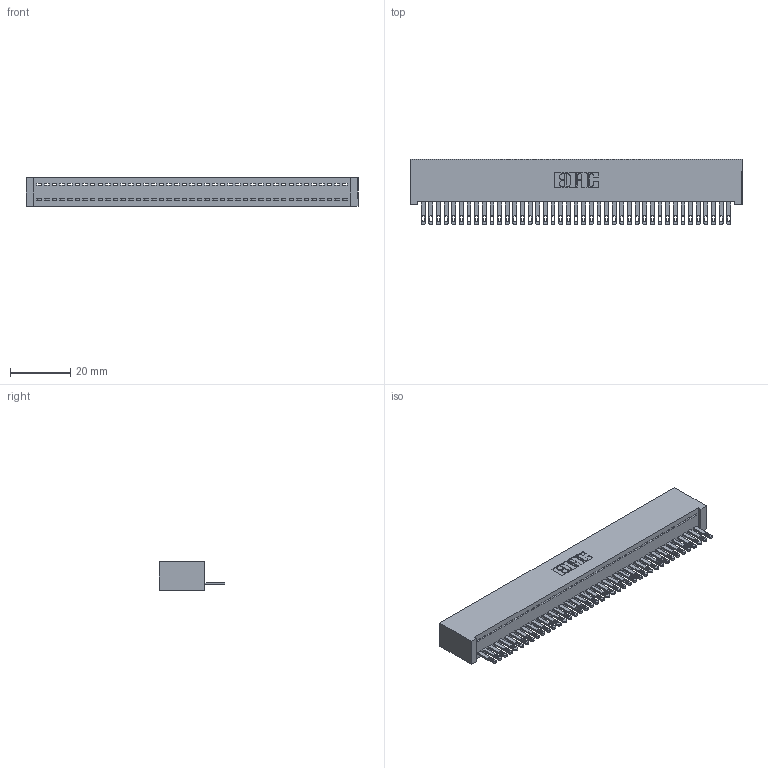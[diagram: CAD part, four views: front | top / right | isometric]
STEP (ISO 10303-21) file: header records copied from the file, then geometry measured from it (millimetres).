
FILE_DESCRIPTION (( 'STEP AP203' ), '1' );
FILE_NAME ('342-041-500-101.STEP', '2019-10-02T17:11:23', ( '' ), ( '' ), 'SwSTEP 2.0', 'SolidWorks 2016', '' );
FILE_SCHEMA (( 'CONFIG_CONTROL_DESIGN' ));
Length unit declared in the file: inch
Products named in the file (3): 342 Part_Lugless; 345-292-001_345-293-100; 342-041-500-101
Assembly tree (42 placements, depth 2):
  342-041-500-101
    342 Part_Lugless
    345-292-001_345-293-100  x41
Bounding box: 110.39 x 21.85 x 9.4 mm (x, y, z)
Volume: 10109.5 mm3; surface area: 15230.7 mm2
Topology: 42 solids, 42 shells, 2316 faces, 7163 edges, 4774 vertices
Faces by surface type: plane 1538, cylinder 778
Entity records: 24715 total; most frequent: CARTESIAN_POINT 4269, ORIENTED_EDGE 4246, DIRECTION 3597, EDGE_CURVE 2123, VECTOR 1999, LINE 1999, VERTEX_POINT 1414, AXIS2_PLACEMENT_3D 799
